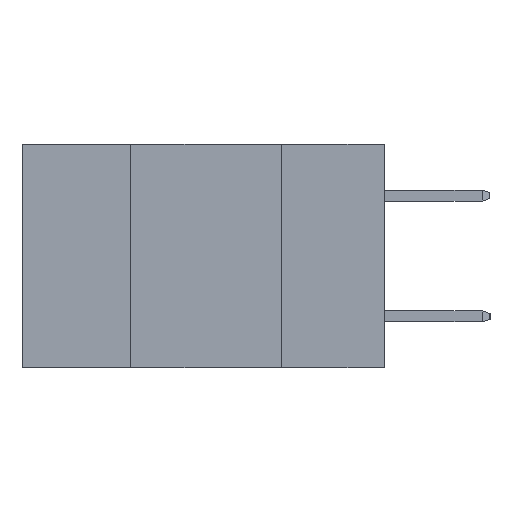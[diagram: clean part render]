
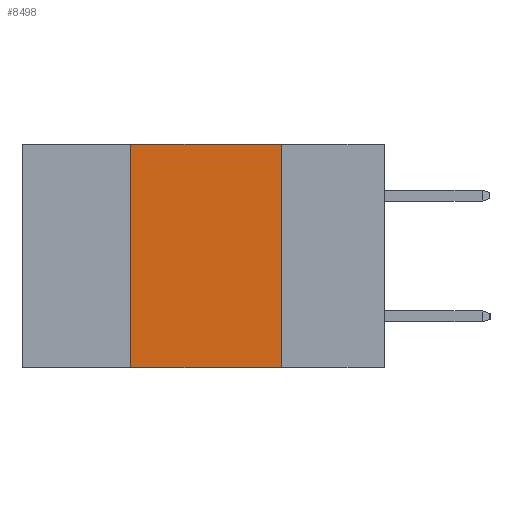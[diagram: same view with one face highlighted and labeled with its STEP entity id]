
A CAD part, left-side view. The second image highlights one B-rep face of the part: STEP entity #8498.
In plain terms, the highlighted planar face has unit normal (-1, 0, 0).
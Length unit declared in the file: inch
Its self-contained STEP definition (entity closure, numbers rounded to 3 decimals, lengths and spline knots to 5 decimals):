
#136 = ORIENTED_EDGE ( 'NONE', *, *, #4466, .F. ) ;
#577 = EDGE_LOOP ( 'NONE', ( #1904, #4369, #136, #2428 ) ) ;
#864 = DIRECTION ( 'NONE',  ( 1., 0., 0. ) ) ;
#1081 = FACE_OUTER_BOUND ( 'NONE', #577, .T. ) ;
#1151 = CARTESIAN_POINT ( 'NONE',  ( 0., 0.42, -0.37 ) ) ;
#1904 = ORIENTED_EDGE ( 'NONE', *, *, #3450, .F. ) ;
#2231 = VECTOR ( 'NONE', #10104, 39.37008 ) ;
#2428 = ORIENTED_EDGE ( 'NONE', *, *, #6353, .T. ) ;
#2487 = LINE ( 'NONE', #3362, #2231 ) ;
#2539 = CARTESIAN_POINT ( 'NONE',  ( 0., 0.6, 0. ) ) ;
#2725 = CARTESIAN_POINT ( 'NONE',  ( 0., 0.42, 0. ) ) ;
#3003 = CARTESIAN_POINT ( 'NONE',  ( 0., 0.17, -0.37 ) ) ;
#3362 = CARTESIAN_POINT ( 'NONE',  ( 0., 0.6, 0. ) ) ;
#3450 = EDGE_CURVE ( 'NONE', #10871, #8739, #8235, .T. ) ;
#4199 = PLANE ( 'NONE',  #10123 ) ;
#4263 = DIRECTION ( 'NONE',  ( 0., 0., -1. ) ) ;
#4369 = ORIENTED_EDGE ( 'NONE', *, *, #4738, .F. ) ;
#4466 = EDGE_CURVE ( 'NONE', #10064, #7634, #5063, .T. ) ;
#4721 = DIRECTION ( 'NONE',  ( 0., -1., 0. ) ) ;
#4738 = EDGE_CURVE ( 'NONE', #7634, #10871, #2487, .T. ) ;
#5063 = LINE ( 'NONE', #8907, #9381 ) ;
#5154 = VECTOR ( 'NONE', #4721, 39.37008 ) ;
#6353 = EDGE_CURVE ( 'NONE', #10064, #8739, #7462, .T. ) ;
#6716 = DIRECTION ( 'NONE',  ( 0., 0., -1. ) ) ;
#7272 = CARTESIAN_POINT ( 'NONE',  ( 0., 0.6, -0.37 ) ) ;
#7462 = LINE ( 'NONE', #7272, #5154 ) ;
#7634 = VERTEX_POINT ( 'NONE', #2725 ) ;
#8235 = LINE ( 'NONE', #3003, #10434 ) ;
#8498 = ADVANCED_FACE ( 'NONE', ( #1081 ), #4199, .F. ) ;
#8739 = VERTEX_POINT ( 'NONE', #10464 ) ;
#8907 = CARTESIAN_POINT ( 'NONE',  ( 0., 0.42, -0.37 ) ) ;
#9381 = VECTOR ( 'NONE', #9727, 39.37008 ) ;
#9727 = DIRECTION ( 'NONE',  ( 0., 0., 1. ) ) ;
#9922 = CARTESIAN_POINT ( 'NONE',  ( 0., 0.17, 0. ) ) ;
#10064 = VERTEX_POINT ( 'NONE', #1151 ) ;
#10104 = DIRECTION ( 'NONE',  ( 0., -1., 0. ) ) ;
#10123 = AXIS2_PLACEMENT_3D ( 'NONE', #2539, #864, #6716 ) ;
#10434 = VECTOR ( 'NONE', #4263, 39.37008 ) ;
#10464 = CARTESIAN_POINT ( 'NONE',  ( 0., 0.17, -0.37 ) ) ;
#10871 = VERTEX_POINT ( 'NONE', #9922 ) ;
